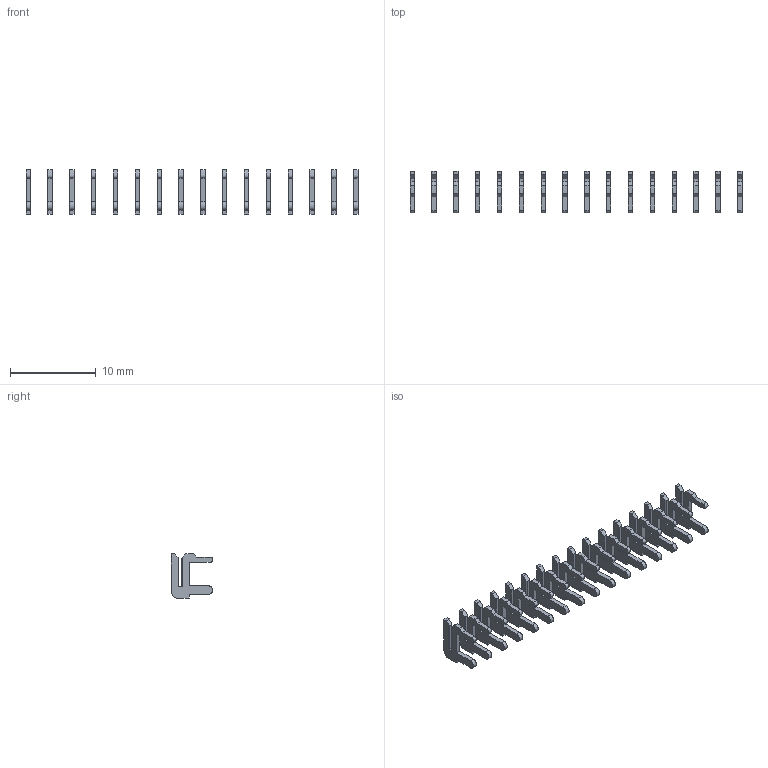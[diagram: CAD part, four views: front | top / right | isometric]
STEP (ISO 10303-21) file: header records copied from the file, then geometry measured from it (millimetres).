
FILE_DESCRIPTION (( 'STEP AP203' ), '1' );
FILE_NAME ('105-016-208-100.STEP', '2020-04-07T22:46:04', ( '' ), ( '' ), 'SwSTEP 2.0', 'SolidWorks 2016', '' );
FILE_SCHEMA (( 'CONFIG_CONTROL_DESIGN' ));
Length unit declared in the file: inch
Products named in the file (2): 105-016-208-100; 100-290-001_100-290-208
Assembly tree (16 placements, depth 2):
  105-016-208-100
    100-290-001_100-290-208  x16
Bounding box: 38.61 x 4.83 x 5.17 mm (x, y, z)
Volume: 110.1 mm3; surface area: 679.9 mm2
Topology: 16 solids, 16 shells, 400 faces, 1104 edges, 736 vertices
Faces by surface type: plane 352, cylinder 48
Entity records: 1469 total; most frequent: DIRECTION 163, CARTESIAN_POINT 159, ORIENTED_EDGE 138, EDGE_CURVE 69, LINE 63, VECTOR 63, AXIS2_PLACEMENT_3D 50, VERTEX_POINT 46
